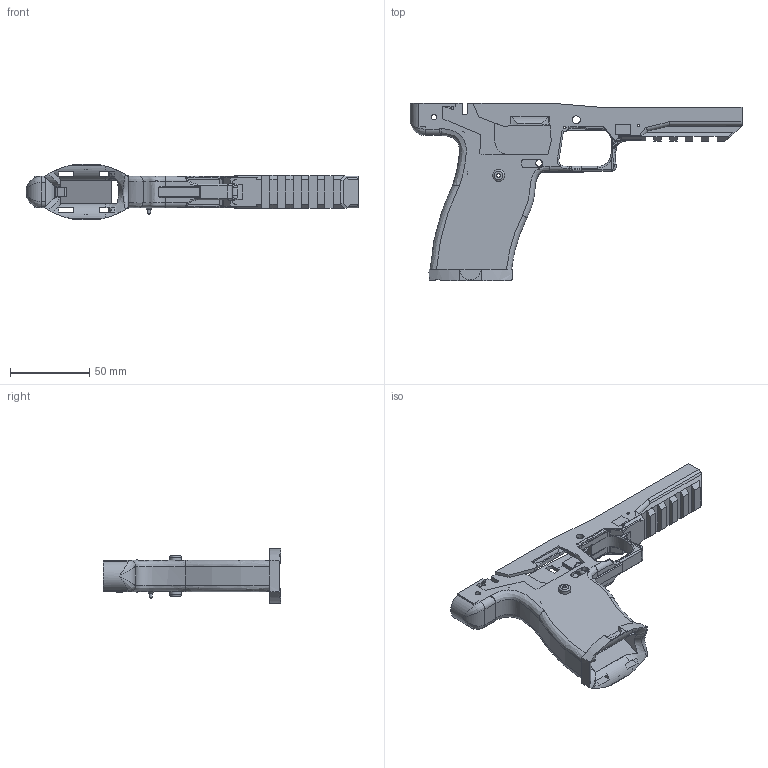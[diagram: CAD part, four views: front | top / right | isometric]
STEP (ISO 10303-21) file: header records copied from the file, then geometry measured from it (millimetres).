
FILE_DESCRIPTION(/* description */ (''),/* implementation_level */ '2;1');
FILE_NAME(/* name */ 'Big-Point Final v1.step',/* time_stamp */ '2020-10-31T21:36:17-04:00',/* author */ (''),/* organization */ (''),/* preprocessor_version */ 'ST-DEVELOPER v18.1',/* originating_system */ 'Autodesk Translation Framework v9.3.0.1241',/* authorisation */ '');
FILE_SCHEMA (('AUTOMOTIVE_DESIGN { 1 0 10303 214 3 1 1 }'));
Length unit declared in the file: millimetre
Products named in the file (1): Big-Point Final
Bounding box: 210 x 112.5 x 35 mm (x, y, z)
Volume: 96898.1 mm3; surface area: 48146.1 mm2
Topology: 1 solids, 2 shells, 502 faces, 1467 edges, 957 vertices
Faces by surface type: plane 294, cylinder 102, bspline 94, torus 10, cone 2
Full cylindrical faces by diameter (mm): 1.5 x5, 1.75 x1, 2 x1, 2.4 x2, 3 x4, 3.5 x2, 3.7 x1, 4 x1, 5 x2, 6.5 x1, 6.75 x1, 7.5 x2
Entity records: 24858 total; most frequent: CARTESIAN_POINT 12198, ORIENTED_EDGE 2910, DIRECTION 2245, EDGE_CURVE 1455, VERTEX_POINT 957, LINE 869, VECTOR 869, AXIS2_PLACEMENT_3D 688
